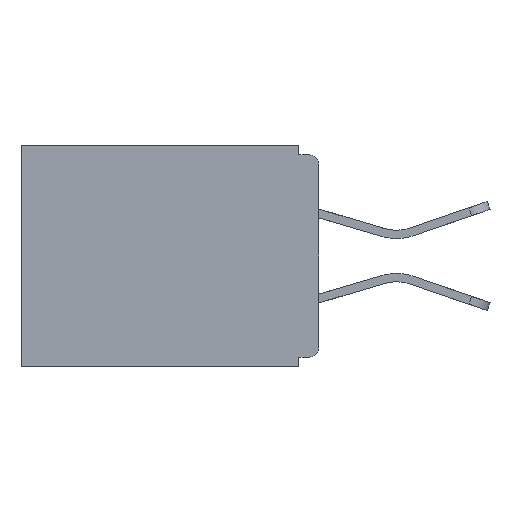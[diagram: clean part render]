
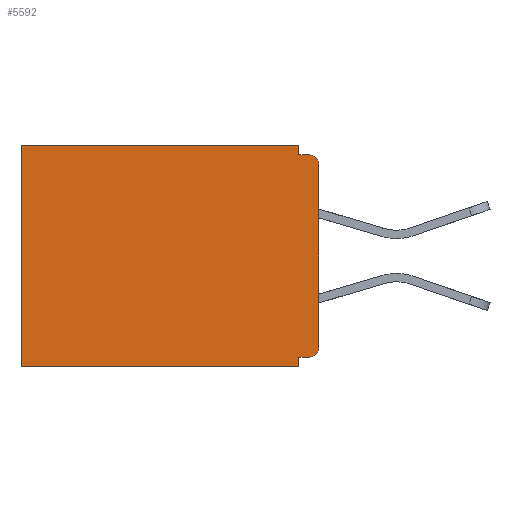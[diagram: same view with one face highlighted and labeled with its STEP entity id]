
A CAD part, left-side view. The second image highlights one B-rep face of the part: STEP entity #5592.
In plain terms, the highlighted planar face has unit normal (-1, 0, 0).
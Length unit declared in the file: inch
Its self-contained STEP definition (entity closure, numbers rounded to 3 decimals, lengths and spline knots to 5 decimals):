
#472 = EDGE_CURVE ( 'NONE', #3089, #8108, #8646, .T. ) ;
#504 = VERTEX_POINT ( 'NONE', #17414 ) ;
#649 = AXIS2_PLACEMENT_3D ( 'NONE', #17326, #9984, #21050 ) ;
#872 = VERTEX_POINT ( 'NONE', #4874 ) ;
#1100 = PLANE ( 'NONE',  #22642 ) ;
#1768 = VECTOR ( 'NONE', #16683, 39.37008 ) ;
#2112 = CARTESIAN_POINT ( 'NONE',  ( 0.298, 0., -0.313 ) ) ;
#2137 = EDGE_CURVE ( 'NONE', #17755, #872, #12730, .T. ) ;
#2271 = CARTESIAN_POINT ( 'NONE',  ( 0.298, 0.031, -0.343 ) ) ;
#2559 = LINE ( 'NONE', #2271, #15414 ) ;
#2865 = ORIENTED_EDGE ( 'NONE', *, *, #13942, .F. ) ;
#2906 = CARTESIAN_POINT ( 'NONE',  ( 0.298, 0.031, -0.343 ) ) ;
#3010 = CARTESIAN_POINT ( 'NONE',  ( 0.298, 0., 0. ) ) ;
#3031 = ORIENTED_EDGE ( 'NONE', *, *, #20104, .F. ) ;
#3089 = VERTEX_POINT ( 'NONE', #8234 ) ;
#3502 = ORIENTED_EDGE ( 'NONE', *, *, #5198, .F. ) ;
#3739 = ORIENTED_EDGE ( 'NONE', *, *, #18519, .F. ) ;
#3750 = DIRECTION ( 'NONE',  ( 0., 1., 0. ) ) ;
#3849 = VERTEX_POINT ( 'NONE', #6827 ) ;
#3916 = ORIENTED_EDGE ( 'NONE', *, *, #12196, .T. ) ;
#4357 = CIRCLE ( 'NONE', #14956, 0.015 ) ;
#4564 = EDGE_CURVE ( 'NONE', #17755, #16705, #2559, .T. ) ;
#4704 = CARTESIAN_POINT ( 'NONE',  ( 0.298, 0.031, -0.015 ) ) ;
#4874 = CARTESIAN_POINT ( 'NONE',  ( 0.298, 0.46, 0. ) ) ;
#5038 = VECTOR ( 'NONE', #18935, 39.37008 ) ;
#5113 = LINE ( 'NONE', #18059, #17095 ) ;
#5198 = EDGE_CURVE ( 'NONE', #19803, #504, #23445, .T. ) ;
#5592 = ADVANCED_FACE ( 'NONE', ( #9640 ), #1100, .F. ) ;
#6827 = CARTESIAN_POINT ( 'NONE',  ( 0.298, 0.031, -0.328 ) ) ;
#7108 = VERTEX_POINT ( 'NONE', #2112 ) ;
#8108 = VERTEX_POINT ( 'NONE', #12216 ) ;
#8234 = CARTESIAN_POINT ( 'NONE',  ( 0.298, 0., -0.03 ) ) ;
#8646 = CIRCLE ( 'NONE', #649, 0.015 ) ;
#9386 = CARTESIAN_POINT ( 'NONE',  ( 0.298, 0.031, -0.343 ) ) ;
#9640 = FACE_OUTER_BOUND ( 'NONE', #20596, .T. ) ;
#9978 = CARTESIAN_POINT ( 'NONE',  ( 0.298, 0., 0. ) ) ;
#9984 = DIRECTION ( 'NONE',  ( -1., 0., 0. ) ) ;
#10440 = LINE ( 'NONE', #15172, #5038 ) ;
#10467 = VERTEX_POINT ( 'NONE', #18664 ) ;
#11108 = VECTOR ( 'NONE', #3750, 39.37008 ) ;
#11335 = LINE ( 'NONE', #14618, #12513 ) ;
#12084 = DIRECTION ( 'NONE',  ( 0., 0., -1. ) ) ;
#12196 = EDGE_CURVE ( 'NONE', #872, #504, #10440, .T. ) ;
#12216 = CARTESIAN_POINT ( 'NONE',  ( 0.298, 0.015, -0.015 ) ) ;
#12513 = VECTOR ( 'NONE', #14538, 39.37008 ) ;
#12730 = LINE ( 'NONE', #9978, #14420 ) ;
#12888 = CARTESIAN_POINT ( 'NONE',  ( 0.298, 0., -0.343 ) ) ;
#13299 = DIRECTION ( 'NONE',  ( 0., 0., -1. ) ) ;
#13423 = ORIENTED_EDGE ( 'NONE', *, *, #19516, .T. ) ;
#13688 = ORIENTED_EDGE ( 'NONE', *, *, #472, .T. ) ;
#13942 = EDGE_CURVE ( 'NONE', #16705, #8108, #20444, .T. ) ;
#14014 = ORIENTED_EDGE ( 'NONE', *, *, #2137, .T. ) ;
#14420 = VECTOR ( 'NONE', #22980, 39.37008 ) ;
#14538 = DIRECTION ( 'NONE',  ( 0., 0., -1. ) ) ;
#14618 = CARTESIAN_POINT ( 'NONE',  ( 0.298, 0., 0. ) ) ;
#14661 = ORIENTED_EDGE ( 'NONE', *, *, #4564, .F. ) ;
#14956 = AXIS2_PLACEMENT_3D ( 'NONE', #15486, #19258, #12084 ) ;
#15172 = CARTESIAN_POINT ( 'NONE',  ( 0.298, 0.46, 0. ) ) ;
#15414 = VECTOR ( 'NONE', #13299, 39.37008 ) ;
#15486 = CARTESIAN_POINT ( 'NONE',  ( 0.298, 0.015, -0.313 ) ) ;
#15532 = EDGE_CURVE ( 'NONE', #3849, #19803, #17459, .T. ) ;
#16683 = DIRECTION ( 'NONE',  ( 0., 0., -1. ) ) ;
#16705 = VERTEX_POINT ( 'NONE', #4704 ) ;
#17095 = VECTOR ( 'NONE', #21693, 39.37008 ) ;
#17227 = ORIENTED_EDGE ( 'NONE', *, *, #15532, .F. ) ;
#17326 = CARTESIAN_POINT ( 'NONE',  ( 0.298, 0.015, -0.03 ) ) ;
#17414 = CARTESIAN_POINT ( 'NONE',  ( 0.298, 0.46, -0.343 ) ) ;
#17459 = LINE ( 'NONE', #9386, #1768 ) ;
#17537 = DIRECTION ( 'NONE',  ( 0., -1., 0. ) ) ;
#17612 = DIRECTION ( 'NONE',  ( 1., 0., 0. ) ) ;
#17755 = VERTEX_POINT ( 'NONE', #23651 ) ;
#17788 = DIRECTION ( 'NONE',  ( 0., 0., -1. ) ) ;
#18059 = CARTESIAN_POINT ( 'NONE',  ( 0.298, 0., -0.328 ) ) ;
#18519 = EDGE_CURVE ( 'NONE', #3089, #7108, #11335, .T. ) ;
#18664 = CARTESIAN_POINT ( 'NONE',  ( 0.298, 0.015, -0.328 ) ) ;
#18935 = DIRECTION ( 'NONE',  ( 0., 0., -1. ) ) ;
#19236 = CARTESIAN_POINT ( 'NONE',  ( 0.298, 0., -0.015 ) ) ;
#19258 = DIRECTION ( 'NONE',  ( -1., 0., 0. ) ) ;
#19516 = EDGE_CURVE ( 'NONE', #10467, #7108, #4357, .T. ) ;
#19803 = VERTEX_POINT ( 'NONE', #2906 ) ;
#20104 = EDGE_CURVE ( 'NONE', #10467, #3849, #5113, .T. ) ;
#20444 = LINE ( 'NONE', #19236, #20744 ) ;
#20596 = EDGE_LOOP ( 'NONE', ( #13688, #2865, #14661, #14014, #3916, #3502, #17227, #3031, #13423, #3739 ) ) ;
#20744 = VECTOR ( 'NONE', #17537, 39.37008 ) ;
#21050 = DIRECTION ( 'NONE',  ( 0., 0., -1. ) ) ;
#21693 = DIRECTION ( 'NONE',  ( 0., 1., 0. ) ) ;
#22642 = AXIS2_PLACEMENT_3D ( 'NONE', #3010, #17612, #17788 ) ;
#22980 = DIRECTION ( 'NONE',  ( 0., 1., 0. ) ) ;
#23445 = LINE ( 'NONE', #12888, #11108 ) ;
#23651 = CARTESIAN_POINT ( 'NONE',  ( 0.298, 0.031, 0. ) ) ;
